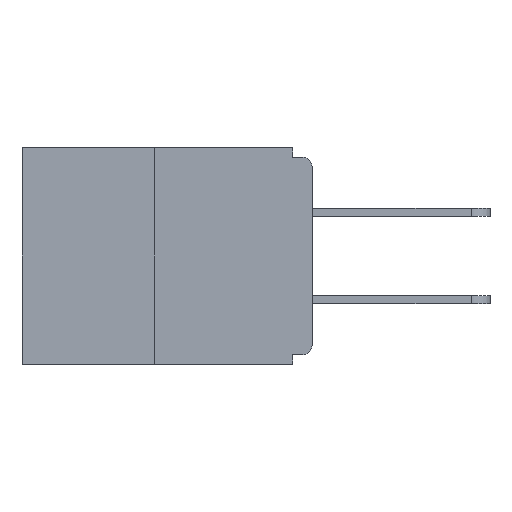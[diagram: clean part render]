
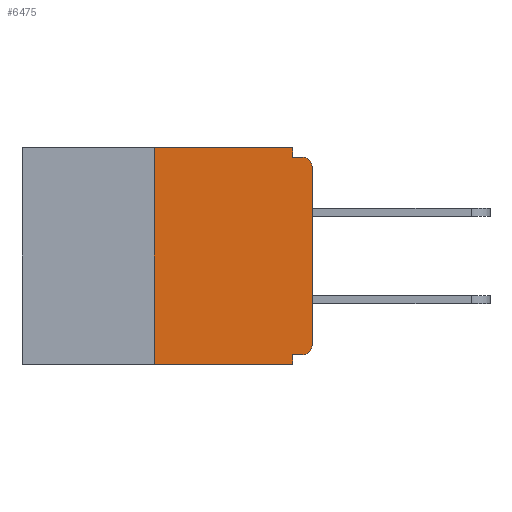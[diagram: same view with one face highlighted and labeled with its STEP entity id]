
A CAD part, left-side view. The second image highlights one B-rep face of the part: STEP entity #6475.
In plain terms, the highlighted planar face has unit normal (-1, 0, 0).
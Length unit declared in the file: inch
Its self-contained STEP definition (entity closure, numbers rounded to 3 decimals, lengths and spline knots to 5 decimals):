
#112 = EDGE_CURVE ( 'NONE', #6178, #12850, #15179, .T. ) ;
#211 = EDGE_CURVE ( 'NONE', #741, #7083, #2423, .T. ) ;
#225 = VECTOR ( 'NONE', #8213, 39.37008 ) ;
#394 = EDGE_CURVE ( 'NONE', #8535, #8659, #4824, .T. ) ;
#429 = DIRECTION ( 'NONE',  ( 0., -1., 0. ) ) ;
#741 = VERTEX_POINT ( 'NONE', #2343 ) ;
#1012 = VECTOR ( 'NONE', #429, 39.37008 ) ;
#1109 = VECTOR ( 'NONE', #1220, 39.37008 ) ;
#1220 = DIRECTION ( 'NONE',  ( 0., 0., 1. ) ) ;
#1239 = FACE_OUTER_BOUND ( 'NONE', #5889, .T. ) ;
#1311 = CARTESIAN_POINT ( 'NONE',  ( 0., 0., -0.015 ) ) ;
#1449 = CARTESIAN_POINT ( 'NONE',  ( 0., 0.015, -0.313 ) ) ;
#1744 = ORIENTED_EDGE ( 'NONE', *, *, #3962, .T. ) ;
#1965 = DIRECTION ( 'NONE',  ( 0., 0., -1. ) ) ;
#2204 = DIRECTION ( 'NONE',  ( 0., 0., -1. ) ) ;
#2343 = CARTESIAN_POINT ( 'NONE',  ( 0., 0.031, -0.328 ) ) ;
#2384 = CARTESIAN_POINT ( 'NONE',  ( 0., 0.25, 0. ) ) ;
#2423 = LINE ( 'NONE', #3509, #17336 ) ;
#2554 = CARTESIAN_POINT ( 'NONE',  ( 0., 0., -0.03 ) ) ;
#2572 = DIRECTION ( 'NONE',  ( 0., 1., 0. ) ) ;
#2680 = CARTESIAN_POINT ( 'NONE',  ( 0., 0.031, 0. ) ) ;
#3032 = ORIENTED_EDGE ( 'NONE', *, *, #12999, .T. ) ;
#3409 = EDGE_CURVE ( 'NONE', #4848, #4985, #16246, .T. ) ;
#3509 = CARTESIAN_POINT ( 'NONE',  ( 0., 0.031, -0.343 ) ) ;
#3546 = AXIS2_PLACEMENT_3D ( 'NONE', #1449, #11253, #15527 ) ;
#3630 = ORIENTED_EDGE ( 'NONE', *, *, #15779, .F. ) ;
#3962 = EDGE_CURVE ( 'NONE', #4118, #4848, #14103, .T. ) ;
#4095 = LINE ( 'NONE', #6056, #1012 ) ;
#4118 = VERTEX_POINT ( 'NONE', #9875 ) ;
#4627 = CARTESIAN_POINT ( 'NONE',  ( 0., 0.015, -0.015 ) ) ;
#4659 = ORIENTED_EDGE ( 'NONE', *, *, #3409, .T. ) ;
#4784 = CARTESIAN_POINT ( 'NONE',  ( 0., 0.031, 0. ) ) ;
#4787 = DIRECTION ( 'NONE',  ( -1., 0., 0. ) ) ;
#4824 = LINE ( 'NONE', #2384, #1109 ) ;
#4848 = VERTEX_POINT ( 'NONE', #2554 ) ;
#4907 = AXIS2_PLACEMENT_3D ( 'NONE', #14320, #4787, #6104 ) ;
#4985 = VERTEX_POINT ( 'NONE', #4627 ) ;
#5003 = VERTEX_POINT ( 'NONE', #14285 ) ;
#5862 = CARTESIAN_POINT ( 'NONE',  ( 0., 0.031, -0.343 ) ) ;
#5889 = EDGE_LOOP ( 'NONE', ( #15123, #6930, #8759, #11652, #10606, #3032, #1744, #4659, #3630, #14107 ) ) ;
#6056 = CARTESIAN_POINT ( 'NONE',  ( 0., 0.46, -0.343 ) ) ;
#6104 = DIRECTION ( 'NONE',  ( 0., 0., -1. ) ) ;
#6177 = VECTOR ( 'NONE', #2572, 39.37008 ) ;
#6178 = VERTEX_POINT ( 'NONE', #2680 ) ;
#6475 = ADVANCED_FACE ( 'NONE', ( #1239 ), #15942, .F. ) ;
#6930 = ORIENTED_EDGE ( 'NONE', *, *, #394, .F. ) ;
#7040 = CARTESIAN_POINT ( 'NONE',  ( 0., 0.25, -0.343 ) ) ;
#7083 = VERTEX_POINT ( 'NONE', #5862 ) ;
#7791 = DIRECTION ( 'NONE',  ( 1., 0., 0. ) ) ;
#8213 = DIRECTION ( 'NONE',  ( 0., -1., 0. ) ) ;
#8460 = DIRECTION ( 'NONE',  ( 0., -1., 0. ) ) ;
#8535 = VERTEX_POINT ( 'NONE', #7040 ) ;
#8659 = VERTEX_POINT ( 'NONE', #11641 ) ;
#8759 = ORIENTED_EDGE ( 'NONE', *, *, #14085, .T. ) ;
#9490 = EDGE_CURVE ( 'NONE', #5003, #741, #16988, .T. ) ;
#9624 = CARTESIAN_POINT ( 'NONE',  ( 0., 0.46, 0. ) ) ;
#9870 = VECTOR ( 'NONE', #8460, 39.37008 ) ;
#9875 = CARTESIAN_POINT ( 'NONE',  ( 0., 0., -0.313 ) ) ;
#10421 = DIRECTION ( 'NONE',  ( 0., 0., 1. ) ) ;
#10509 = LINE ( 'NONE', #1311, #9870 ) ;
#10606 = ORIENTED_EDGE ( 'NONE', *, *, #9490, .F. ) ;
#10788 = CIRCLE ( 'NONE', #3546, 0.015 ) ;
#11253 = DIRECTION ( 'NONE',  ( -1., 0., 0. ) ) ;
#11641 = CARTESIAN_POINT ( 'NONE',  ( 0., 0.25, 0. ) ) ;
#11652 = ORIENTED_EDGE ( 'NONE', *, *, #211, .F. ) ;
#11701 = AXIS2_PLACEMENT_3D ( 'NONE', #13292, #7791, #14908 ) ;
#12451 = EDGE_CURVE ( 'NONE', #8659, #6178, #15345, .T. ) ;
#12593 = VECTOR ( 'NONE', #10421, 39.37008 ) ;
#12850 = VERTEX_POINT ( 'NONE', #17788 ) ;
#12999 = EDGE_CURVE ( 'NONE', #5003, #4118, #10788, .T. ) ;
#13231 = CARTESIAN_POINT ( 'NONE',  ( 0., 0., 0. ) ) ;
#13292 = CARTESIAN_POINT ( 'NONE',  ( 0., 0.46, 0. ) ) ;
#14085 = EDGE_CURVE ( 'NONE', #8535, #7083, #4095, .T. ) ;
#14103 = LINE ( 'NONE', #13231, #12593 ) ;
#14107 = ORIENTED_EDGE ( 'NONE', *, *, #112, .F. ) ;
#14285 = CARTESIAN_POINT ( 'NONE',  ( 0., 0.015, -0.328 ) ) ;
#14320 = CARTESIAN_POINT ( 'NONE',  ( 0., 0.015, -0.03 ) ) ;
#14908 = DIRECTION ( 'NONE',  ( 0., 0., -1. ) ) ;
#15123 = ORIENTED_EDGE ( 'NONE', *, *, #12451, .F. ) ;
#15179 = LINE ( 'NONE', #4784, #17747 ) ;
#15345 = LINE ( 'NONE', #9624, #225 ) ;
#15527 = DIRECTION ( 'NONE',  ( 0., 0., -1. ) ) ;
#15779 = EDGE_CURVE ( 'NONE', #12850, #4985, #10509, .T. ) ;
#15942 = PLANE ( 'NONE',  #11701 ) ;
#16246 = CIRCLE ( 'NONE', #4907, 0.015 ) ;
#16988 = LINE ( 'NONE', #17774, #6177 ) ;
#17336 = VECTOR ( 'NONE', #2204, 39.37008 ) ;
#17747 = VECTOR ( 'NONE', #1965, 39.37008 ) ;
#17774 = CARTESIAN_POINT ( 'NONE',  ( 0., 0., -0.328 ) ) ;
#17788 = CARTESIAN_POINT ( 'NONE',  ( 0., 0.031, -0.015 ) ) ;
